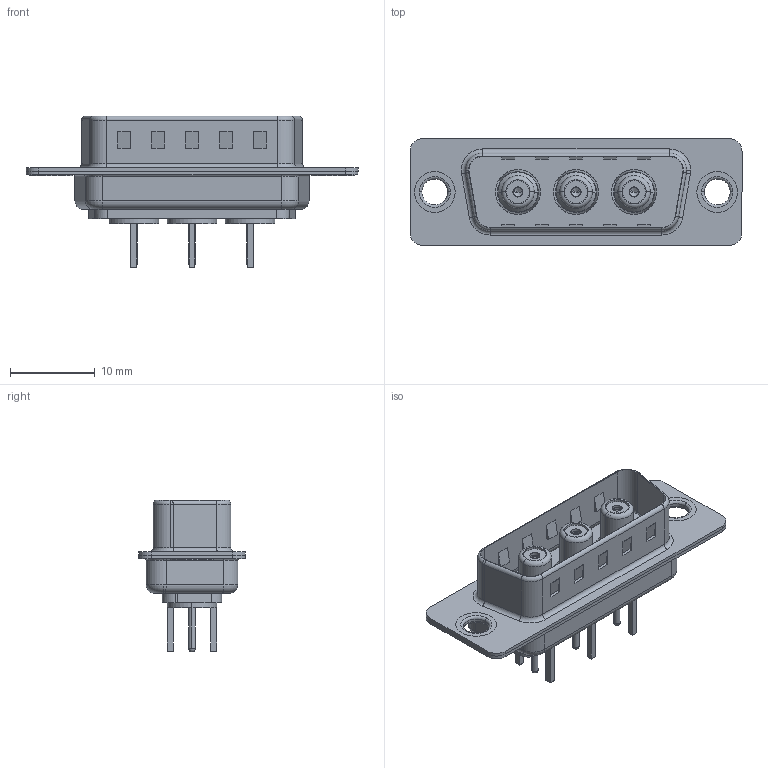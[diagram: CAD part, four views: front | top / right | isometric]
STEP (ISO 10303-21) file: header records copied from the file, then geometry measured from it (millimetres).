
FILE_DESCRIPTION (( 'STEP AP203' ), '1' );
FILE_NAME ('627-3W3-224-7T1.STEP', '2019-05-24T15:49:31', ( '' ), ( '' ), 'SwSTEP 2.0', 'SolidWorks 2016', '' );
FILE_SCHEMA (( 'CONFIG_CONTROL_DESIGN' ));
Length unit declared in the file: millimetre
Products named in the file (11): Locking Collar; Socket_Str; 627Combo Housing_3W3; Co-Ax Jack Assy_S; 627Combo Shell Rear_15 Contacts; 627Combo Shell Front_15 Contacts; 627-3W3-224-7T1; 627Combo Thru Hole Rivet; Co-Ax Jack_Straight PC Tail; Insulator Socket; Insulator Socket 2
Assembly tree (13 placements, depth 3):
  627-3W3-224-7T1
    627Combo Housing_3W3
    627Combo Shell Rear_15 Contacts
    627Combo Shell Front_15 Contacts
    627Combo Thru Hole Rivet  x2
    Co-Ax Jack Assy_S  x3
      Co-Ax Jack_Straight PC Tail
      Insulator Socket
      Insulator Socket 2
      Locking Collar
      Socket_Str
Bounding box: 39.15 x 12.6 x 17.9 mm (x, y, z)
Volume: 1829.4 mm3; surface area: 5775 mm2
Topology: 20 solids, 20 shells, 647 faces, 1522 edges, 950 vertices
Faces by surface type: plane 280, cylinder 258, torus 70, cone 27, bspline 6, sphere 6
Entity records: 13561 total; most frequent: DIRECTION 2256, CARTESIAN_POINT 2213, ORIENTED_EDGE 2004, EDGE_CURVE 1002, AXIS2_PLACEMENT_3D 851, VERTEX_POINT 630, LINE 554, VECTOR 554
